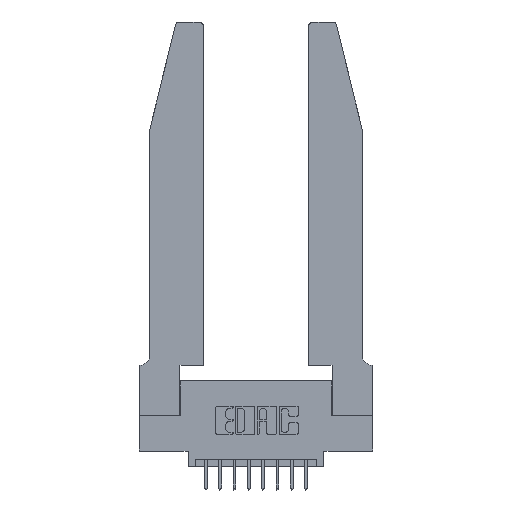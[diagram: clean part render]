
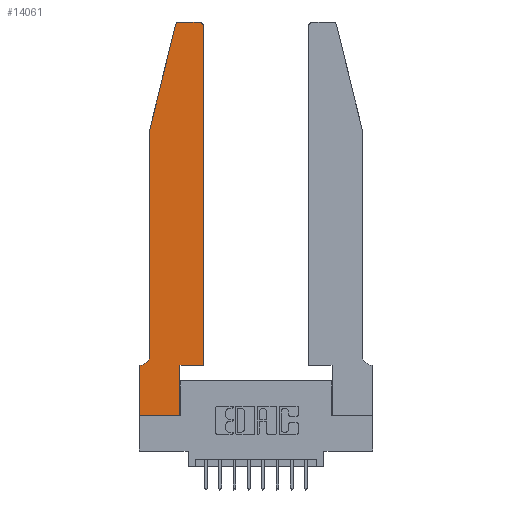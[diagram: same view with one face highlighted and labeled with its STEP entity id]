
A CAD part, top view. The second image highlights one B-rep face of the part: STEP entity #14061.
In plain terms, the highlighted planar face has unit normal (0, 0, 1).
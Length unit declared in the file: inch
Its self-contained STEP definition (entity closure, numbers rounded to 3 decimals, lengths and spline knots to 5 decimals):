
#16 = CARTESIAN_POINT ( 'NONE',  ( 0.0755, 0.42, 0.37 ) ) ;
#109 = EDGE_CURVE ( 'NONE', #8468, #13557, #11006, .T. ) ;
#183 = AXIS2_PLACEMENT_3D ( 'NONE', #1074, #7524, #6366 ) ;
#249 = VECTOR ( 'NONE', #5350, 39.37008 ) ;
#324 = EDGE_CURVE ( 'NONE', #9829, #1346, #7755, .T. ) ;
#338 = DIRECTION ( 'NONE',  ( 0., 0., 1. ) ) ;
#641 = CARTESIAN_POINT ( 'NONE',  ( 0.0755, 0.35, 0.37 ) ) ;
#841 = CIRCLE ( 'NONE', #3877, 0.03 ) ;
#1074 = CARTESIAN_POINT ( 'NONE',  ( 0.0055, 0.42, 0.37 ) ) ;
#1129 = AXIS2_PLACEMENT_3D ( 'NONE', #7777, #7833, #8910 ) ;
#1346 = VERTEX_POINT ( 'NONE', #3884 ) ;
#1454 = ORIENTED_EDGE ( 'NONE', *, *, #324, .T. ) ;
#1459 = CARTESIAN_POINT ( 'NONE',  ( 0.284, 2.72, 0.37 ) ) ;
#1651 = EDGE_CURVE ( 'NONE', #2130, #15779, #5578, .T. ) ;
#1684 = LINE ( 'NONE', #4108, #10877 ) ;
#1871 = CARTESIAN_POINT ( 'NONE',  ( 0.2865, 0., 0.37 ) ) ;
#2130 = VERTEX_POINT ( 'NONE', #15233 ) ;
#2468 = VECTOR ( 'NONE', #8135, 39.37008 ) ;
#2628 = ORIENTED_EDGE ( 'NONE', *, *, #8002, .T. ) ;
#2712 = LINE ( 'NONE', #4056, #249 ) ;
#3193 = LINE ( 'NONE', #11748, #2468 ) ;
#3276 = ORIENTED_EDGE ( 'NONE', *, *, #9490, .T. ) ;
#3315 = VECTOR ( 'NONE', #13755, 39.37008 ) ;
#3563 = CARTESIAN_POINT ( 'NONE',  ( 0.4505, 2.72, 0.37 ) ) ;
#3585 = ORIENTED_EDGE ( 'NONE', *, *, #4830, .T. ) ;
#3614 = AXIS2_PLACEMENT_3D ( 'NONE', #8678, #7924, #4042 ) ;
#3640 = CARTESIAN_POINT ( 'NONE',  ( 0.4505, 0.35, 0.37 ) ) ;
#3845 = LINE ( 'NONE', #5171, #14589 ) ;
#3877 = AXIS2_PLACEMENT_3D ( 'NONE', #1459, #338, #11250 ) ;
#3884 = CARTESIAN_POINT ( 'NONE',  ( 0.284, 2.75, 0.37 ) ) ;
#4042 = DIRECTION ( 'NONE',  ( 1., 0., 0. ) ) ;
#4056 = CARTESIAN_POINT ( 'NONE',  ( 0.0755, 2., 0.37 ) ) ;
#4108 = CARTESIAN_POINT ( 'NONE',  ( 0., 0., 0.37 ) ) ;
#4294 = ORIENTED_EDGE ( 'NONE', *, *, #109, .T. ) ;
#4687 = FACE_OUTER_BOUND ( 'NONE', #9396, .T. ) ;
#4830 = EDGE_CURVE ( 'NONE', #13557, #4956, #11793, .T. ) ;
#4956 = VERTEX_POINT ( 'NONE', #8571 ) ;
#5171 = CARTESIAN_POINT ( 'NONE',  ( 0.4505, 0.35, 0.37 ) ) ;
#5227 = CARTESIAN_POINT ( 'NONE',  ( 0.4505, 0.35, 0.37 ) ) ;
#5350 = DIRECTION ( 'NONE',  ( -0.239, -0.971, 0. ) ) ;
#5578 = LINE ( 'NONE', #9819, #14979 ) ;
#6013 = CARTESIAN_POINT ( 'NONE',  ( 0.4205, 2.75, 0.37 ) ) ;
#6366 = DIRECTION ( 'NONE',  ( -1., 0., 0. ) ) ;
#6446 = ORIENTED_EDGE ( 'NONE', *, *, #7400, .T. ) ;
#6788 = CARTESIAN_POINT ( 'NONE',  ( 0.2605, 2.75, 0.37 ) ) ;
#6839 = DIRECTION ( 'NONE',  ( -1., 0., 0. ) ) ;
#7178 = VECTOR ( 'NONE', #6839, 39.37008 ) ;
#7400 = EDGE_CURVE ( 'NONE', #14065, #13886, #3845, .T. ) ;
#7524 = DIRECTION ( 'NONE',  ( 0., 0., -1. ) ) ;
#7755 = LINE ( 'NONE', #6788, #7178 ) ;
#7777 = CARTESIAN_POINT ( 'NONE',  ( 0.4205, 2.72, 0.37 ) ) ;
#7833 = DIRECTION ( 'NONE',  ( 0., 0., 1. ) ) ;
#7886 = EDGE_CURVE ( 'NONE', #12736, #14065, #11339, .T. ) ;
#7924 = DIRECTION ( 'NONE',  ( 0., 0., 1. ) ) ;
#8002 = EDGE_CURVE ( 'NONE', #14456, #2130, #2712, .T. ) ;
#8135 = DIRECTION ( 'NONE',  ( 0., 1., 0. ) ) ;
#8245 = CARTESIAN_POINT ( 'NONE',  ( 0.25487, 2.72718, 0.37 ) ) ;
#8468 = VERTEX_POINT ( 'NONE', #9840 ) ;
#8571 = CARTESIAN_POINT ( 'NONE',  ( 0., 0., 0.37 ) ) ;
#8590 = ORIENTED_EDGE ( 'NONE', *, *, #1651, .T. ) ;
#8678 = CARTESIAN_POINT ( 'NONE',  ( 0., 0.35, 0.37 ) ) ;
#8910 = DIRECTION ( 'NONE',  ( 1., 0., 0. ) ) ;
#9066 = CARTESIAN_POINT ( 'NONE',  ( 0., 0.35, 0.37 ) ) ;
#9396 = EDGE_LOOP ( 'NONE', ( #1454, #14533, #2628, #8590, #12133, #4294, #3585, #10145, #15515, #11966, #6446, #3276 ) ) ;
#9490 = EDGE_CURVE ( 'NONE', #13886, #9829, #9608, .T. ) ;
#9590 = DIRECTION ( 'NONE',  ( 1., 0., 0. ) ) ;
#9608 = CIRCLE ( 'NONE', #1129, 0.03 ) ;
#9615 = EDGE_CURVE ( 'NONE', #1346, #14456, #841, .T. ) ;
#9677 = VECTOR ( 'NONE', #14690, 39.37008 ) ;
#9801 = CARTESIAN_POINT ( 'NONE',  ( 0., 0., 0.37 ) ) ;
#9819 = CARTESIAN_POINT ( 'NONE',  ( 0.0755, 2., 0.37 ) ) ;
#9829 = VERTEX_POINT ( 'NONE', #6013 ) ;
#9840 = CARTESIAN_POINT ( 'NONE',  ( 0.0055, 0.35, 0.37 ) ) ;
#10145 = ORIENTED_EDGE ( 'NONE', *, *, #13568, .T. ) ;
#10203 = DIRECTION ( 'NONE',  ( 0., 1., 0. ) ) ;
#10409 = CIRCLE ( 'NONE', #183, 0.07 ) ;
#10564 = VECTOR ( 'NONE', #9590, 39.37008 ) ;
#10877 = VECTOR ( 'NONE', #13713, 39.37008 ) ;
#11006 = LINE ( 'NONE', #641, #3315 ) ;
#11011 = DIRECTION ( 'NONE',  ( 0., -1., 0. ) ) ;
#11250 = DIRECTION ( 'NONE',  ( 1., 0., 0. ) ) ;
#11339 = LINE ( 'NONE', #3640, #10564 ) ;
#11361 = CARTESIAN_POINT ( 'NONE',  ( 0.2865, 0.35, 0.37 ) ) ;
#11665 = EDGE_CURVE ( 'NONE', #12856, #12736, #3193, .T. ) ;
#11748 = CARTESIAN_POINT ( 'NONE',  ( 0.2865, 0.35, 0.37 ) ) ;
#11793 = LINE ( 'NONE', #9801, #9677 ) ;
#11966 = ORIENTED_EDGE ( 'NONE', *, *, #7886, .T. ) ;
#12133 = ORIENTED_EDGE ( 'NONE', *, *, #15808, .T. ) ;
#12736 = VERTEX_POINT ( 'NONE', #11361 ) ;
#12856 = VERTEX_POINT ( 'NONE', #1871 ) ;
#13557 = VERTEX_POINT ( 'NONE', #9066 ) ;
#13568 = EDGE_CURVE ( 'NONE', #4956, #12856, #1684, .T. ) ;
#13713 = DIRECTION ( 'NONE',  ( 1., 0., 0. ) ) ;
#13755 = DIRECTION ( 'NONE',  ( -1., 0., 0. ) ) ;
#13886 = VERTEX_POINT ( 'NONE', #3563 ) ;
#14061 = ADVANCED_FACE ( 'NONE', ( #4687 ), #14784, .T. ) ;
#14065 = VERTEX_POINT ( 'NONE', #5227 ) ;
#14456 = VERTEX_POINT ( 'NONE', #8245 ) ;
#14533 = ORIENTED_EDGE ( 'NONE', *, *, #9615, .T. ) ;
#14589 = VECTOR ( 'NONE', #10203, 39.37008 ) ;
#14690 = DIRECTION ( 'NONE',  ( 0., -1., 0. ) ) ;
#14784 = PLANE ( 'NONE',  #3614 ) ;
#14979 = VECTOR ( 'NONE', #11011, 39.37008 ) ;
#15233 = CARTESIAN_POINT ( 'NONE',  ( 0.0755, 2., 0.37 ) ) ;
#15515 = ORIENTED_EDGE ( 'NONE', *, *, #11665, .T. ) ;
#15779 = VERTEX_POINT ( 'NONE', #16 ) ;
#15808 = EDGE_CURVE ( 'NONE', #15779, #8468, #10409, .T. ) ;
